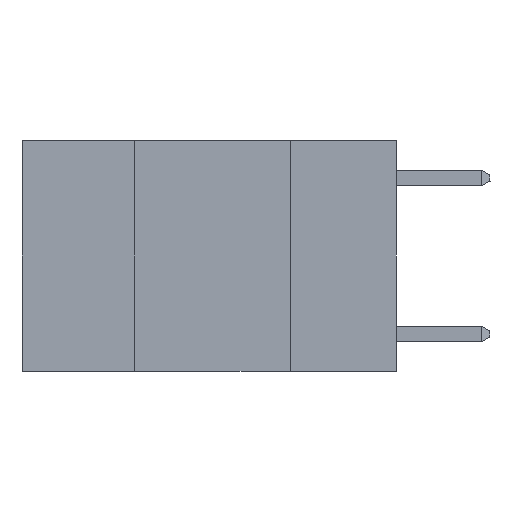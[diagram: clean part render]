
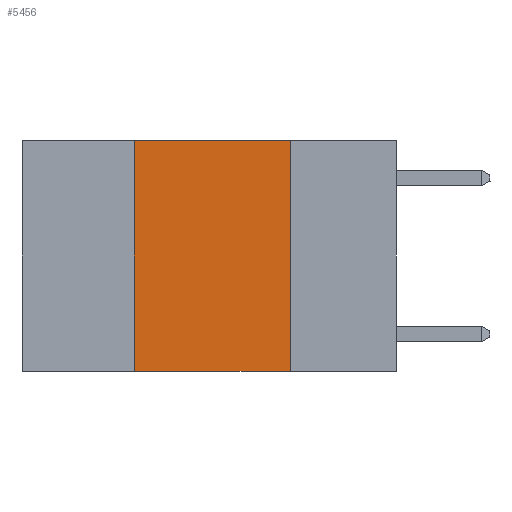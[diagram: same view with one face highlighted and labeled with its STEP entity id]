
A CAD part, left-side view. The second image highlights one B-rep face of the part: STEP entity #5456.
In plain terms, the highlighted planar face has unit normal (-1, 0, 0).
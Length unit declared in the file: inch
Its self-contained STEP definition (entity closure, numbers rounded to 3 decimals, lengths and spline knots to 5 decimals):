
#94 = DIRECTION ( 'NONE',  ( 0., -1., 0. ) ) ;
#129 = LINE ( 'NONE', #5304, #8219 ) ;
#200 = FACE_OUTER_BOUND ( 'NONE', #9050, .T. ) ;
#290 = DIRECTION ( 'NONE',  ( 0., 0., 1. ) ) ;
#462 = DIRECTION ( 'NONE',  ( 0., 0., -1. ) ) ;
#1312 = LINE ( 'NONE', #7529, #7332 ) ;
#1590 = CARTESIAN_POINT ( 'NONE',  ( 0., 0.42, 0. ) ) ;
#1717 = VECTOR ( 'NONE', #94, 39.37008 ) ;
#1968 = LINE ( 'NONE', #4417, #1717 ) ;
#3207 = DIRECTION ( 'NONE',  ( 0., 0., -1. ) ) ;
#3824 = EDGE_CURVE ( 'NONE', #7779, #7020, #1312, .T. ) ;
#3900 = CARTESIAN_POINT ( 'NONE',  ( 0., 0.42, -0.37 ) ) ;
#4127 = ORIENTED_EDGE ( 'NONE', *, *, #9236, .T. ) ;
#4417 = CARTESIAN_POINT ( 'NONE',  ( 0., 0.6, -0.37 ) ) ;
#4589 = LINE ( 'NONE', #4980, #6921 ) ;
#4781 = VERTEX_POINT ( 'NONE', #1590 ) ;
#4980 = CARTESIAN_POINT ( 'NONE',  ( 0., 0.42, 0. ) ) ;
#5304 = CARTESIAN_POINT ( 'NONE',  ( 0., 0.6, 0. ) ) ;
#5436 = AXIS2_PLACEMENT_3D ( 'NONE', #9413, #7892, #3207 ) ;
#5456 = ADVANCED_FACE ( 'NONE', ( #200 ), #5544, .F. ) ;
#5536 = CARTESIAN_POINT ( 'NONE',  ( 0., 0.17, -0.37 ) ) ;
#5544 = PLANE ( 'NONE',  #5436 ) ;
#5717 = ORIENTED_EDGE ( 'NONE', *, *, #9669, .F. ) ;
#5956 = ORIENTED_EDGE ( 'NONE', *, *, #7166, .F. ) ;
#5965 = VERTEX_POINT ( 'NONE', #3900 ) ;
#6921 = VECTOR ( 'NONE', #290, 39.37008 ) ;
#7020 = VERTEX_POINT ( 'NONE', #5536 ) ;
#7166 = EDGE_CURVE ( 'NONE', #5965, #4781, #4589, .T. ) ;
#7332 = VECTOR ( 'NONE', #462, 39.37008 ) ;
#7529 = CARTESIAN_POINT ( 'NONE',  ( 0., 0.17, 0. ) ) ;
#7545 = ORIENTED_EDGE ( 'NONE', *, *, #3824, .F. ) ;
#7779 = VERTEX_POINT ( 'NONE', #8791 ) ;
#7892 = DIRECTION ( 'NONE',  ( 1., 0., 0. ) ) ;
#8219 = VECTOR ( 'NONE', #8372, 39.37008 ) ;
#8372 = DIRECTION ( 'NONE',  ( 0., -1., 0. ) ) ;
#8791 = CARTESIAN_POINT ( 'NONE',  ( 0., 0.17, 0. ) ) ;
#9050 = EDGE_LOOP ( 'NONE', ( #7545, #5717, #5956, #4127 ) ) ;
#9236 = EDGE_CURVE ( 'NONE', #5965, #7020, #1968, .T. ) ;
#9413 = CARTESIAN_POINT ( 'NONE',  ( 0., 0.6, 0. ) ) ;
#9669 = EDGE_CURVE ( 'NONE', #4781, #7779, #129, .T. ) ;
